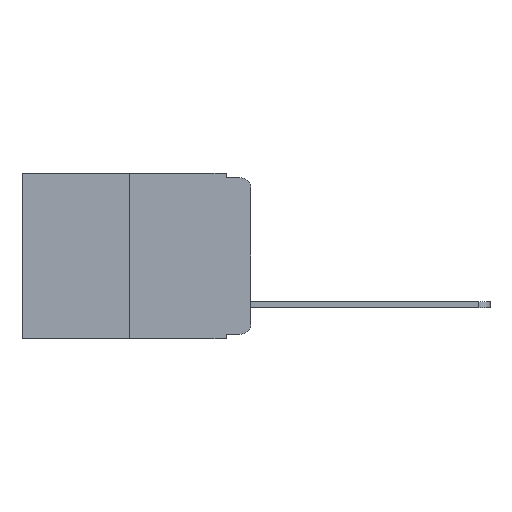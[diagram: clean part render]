
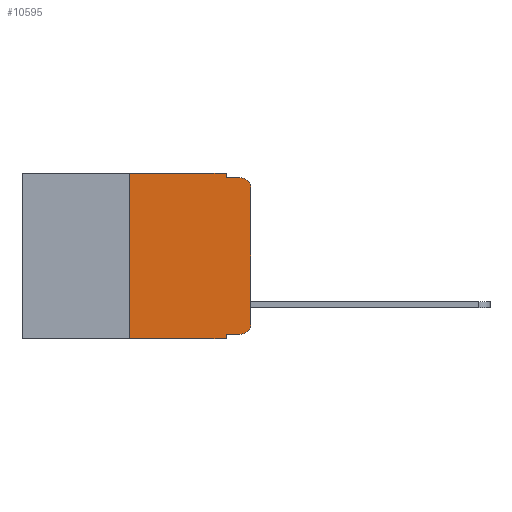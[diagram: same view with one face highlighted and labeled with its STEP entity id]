
A CAD part, left-side view. The second image highlights one B-rep face of the part: STEP entity #10595.
In plain terms, the highlighted planar face has unit normal (-1, 0, 0).
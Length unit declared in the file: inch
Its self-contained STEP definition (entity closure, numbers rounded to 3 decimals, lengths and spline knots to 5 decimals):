
#215 = CIRCLE ( 'NONE', #12082, 0.02 ) ;
#625 = CARTESIAN_POINT ( 'NONE',  ( 0., 0.02, -0.03 ) ) ;
#1014 = VECTOR ( 'NONE', #9177, 39.37008 ) ;
#1016 = CARTESIAN_POINT ( 'NONE',  ( 0., 0.051, -0.343 ) ) ;
#1036 = ORIENTED_EDGE ( 'NONE', *, *, #3050, .T. ) ;
#1070 = ORIENTED_EDGE ( 'NONE', *, *, #10524, .F. ) ;
#1094 = VERTEX_POINT ( 'NONE', #12182 ) ;
#1296 = VERTEX_POINT ( 'NONE', #3679 ) ;
#1349 = AXIS2_PLACEMENT_3D ( 'NONE', #4786, #11981, #3943 ) ;
#1598 = DIRECTION ( 'NONE',  ( 0., 0., -1. ) ) ;
#1734 = VERTEX_POINT ( 'NONE', #9774 ) ;
#1840 = CARTESIAN_POINT ( 'NONE',  ( 0., 0., -0.03 ) ) ;
#2031 = CARTESIAN_POINT ( 'NONE',  ( 0., 0.25, 0. ) ) ;
#2047 = VECTOR ( 'NONE', #7870, 39.37008 ) ;
#2433 = EDGE_CURVE ( 'NONE', #7922, #14541, #15840, .T. ) ;
#2986 = CARTESIAN_POINT ( 'NONE',  ( 0., 0.051, -0.01 ) ) ;
#3050 = EDGE_CURVE ( 'NONE', #1094, #6382, #11726, .T. ) ;
#3128 = VERTEX_POINT ( 'NONE', #5985 ) ;
#3660 = VERTEX_POINT ( 'NONE', #1016 ) ;
#3679 = CARTESIAN_POINT ( 'NONE',  ( 0., 0.02, -0.01 ) ) ;
#3714 = EDGE_CURVE ( 'NONE', #14541, #14164, #4104, .T. ) ;
#3845 = LINE ( 'NONE', #4801, #13199 ) ;
#3943 = DIRECTION ( 'NONE',  ( 0., 0., -1. ) ) ;
#4104 = LINE ( 'NONE', #5399, #11893 ) ;
#4330 = DIRECTION ( 'NONE',  ( -1., 0., 0. ) ) ;
#4376 = CARTESIAN_POINT ( 'NONE',  ( 0., 0., 0. ) ) ;
#4561 = DIRECTION ( 'NONE',  ( 0., -1., 0. ) ) ;
#4786 = CARTESIAN_POINT ( 'NONE',  ( 0., 0.473, 0. ) ) ;
#4801 = CARTESIAN_POINT ( 'NONE',  ( 0., 0.051, 0. ) ) ;
#4833 = ORIENTED_EDGE ( 'NONE', *, *, #2433, .F. ) ;
#5399 = CARTESIAN_POINT ( 'NONE',  ( 0., 0.051, 0. ) ) ;
#5890 = DIRECTION ( 'NONE',  ( 0., 0., -1. ) ) ;
#5968 = EDGE_CURVE ( 'NONE', #8746, #3660, #3845, .T. ) ;
#5985 = CARTESIAN_POINT ( 'NONE',  ( 0., 0.25, -0.343 ) ) ;
#6382 = VERTEX_POINT ( 'NONE', #1840 ) ;
#6638 = AXIS2_PLACEMENT_3D ( 'NONE', #12515, #7379, #16108 ) ;
#6872 = VECTOR ( 'NONE', #4561, 39.37008 ) ;
#6917 = LINE ( 'NONE', #10280, #2047 ) ;
#7094 = CARTESIAN_POINT ( 'NONE',  ( 0., 0.473, 0. ) ) ;
#7379 = DIRECTION ( 'NONE',  ( -1., 0., 0. ) ) ;
#7445 = LINE ( 'NONE', #14098, #12525 ) ;
#7568 = ORIENTED_EDGE ( 'NONE', *, *, #12977, .F. ) ;
#7862 = CARTESIAN_POINT ( 'NONE',  ( 0., 0.25, 0. ) ) ;
#7870 = DIRECTION ( 'NONE',  ( 0., -1., 0. ) ) ;
#7922 = VERTEX_POINT ( 'NONE', #2031 ) ;
#7930 = VECTOR ( 'NONE', #8545, 39.37008 ) ;
#8419 = EDGE_CURVE ( 'NONE', #1734, #1094, #15742, .T. ) ;
#8522 = ORIENTED_EDGE ( 'NONE', *, *, #8419, .T. ) ;
#8545 = DIRECTION ( 'NONE',  ( 0., -1., 0. ) ) ;
#8589 = ORIENTED_EDGE ( 'NONE', *, *, #5968, .F. ) ;
#8746 = VERTEX_POINT ( 'NONE', #14678 ) ;
#8948 = EDGE_LOOP ( 'NONE', ( #1036, #9294, #1070, #12809, #4833, #7568, #10933, #8589, #15335, #8522 ) ) ;
#9177 = DIRECTION ( 'NONE',  ( 0., 0., 1. ) ) ;
#9294 = ORIENTED_EDGE ( 'NONE', *, *, #14126, .T. ) ;
#9774 = CARTESIAN_POINT ( 'NONE',  ( 0., 0.02, -0.333 ) ) ;
#10003 = VECTOR ( 'NONE', #13967, 39.37008 ) ;
#10280 = CARTESIAN_POINT ( 'NONE',  ( 0., 0.051, -0.01 ) ) ;
#10524 = EDGE_CURVE ( 'NONE', #14164, #1296, #6917, .T. ) ;
#10595 = ADVANCED_FACE ( 'NONE', ( #15698 ), #11453, .F. ) ;
#10676 = LINE ( 'NONE', #15976, #7930 ) ;
#10933 = ORIENTED_EDGE ( 'NONE', *, *, #12465, .T. ) ;
#11453 = PLANE ( 'NONE',  #1349 ) ;
#11726 = LINE ( 'NONE', #4376, #1014 ) ;
#11893 = VECTOR ( 'NONE', #1598, 39.37008 ) ;
#11981 = DIRECTION ( 'NONE',  ( 1., 0., 0. ) ) ;
#12082 = AXIS2_PLACEMENT_3D ( 'NONE', #625, #4330, #14282 ) ;
#12182 = CARTESIAN_POINT ( 'NONE',  ( 0., 0., -0.313 ) ) ;
#12465 = EDGE_CURVE ( 'NONE', #3128, #3660, #7445, .T. ) ;
#12515 = CARTESIAN_POINT ( 'NONE',  ( 0., 0.02, -0.313 ) ) ;
#12525 = VECTOR ( 'NONE', #13099, 39.37008 ) ;
#12531 = CARTESIAN_POINT ( 'NONE',  ( 0., 0.051, 0. ) ) ;
#12809 = ORIENTED_EDGE ( 'NONE', *, *, #3714, .F. ) ;
#12977 = EDGE_CURVE ( 'NONE', #3128, #7922, #13569, .T. ) ;
#13099 = DIRECTION ( 'NONE',  ( 0., -1., 0. ) ) ;
#13199 = VECTOR ( 'NONE', #5890, 39.37008 ) ;
#13569 = LINE ( 'NONE', #7862, #10003 ) ;
#13967 = DIRECTION ( 'NONE',  ( 0., 0., 1. ) ) ;
#14098 = CARTESIAN_POINT ( 'NONE',  ( 0., 0.473, -0.343 ) ) ;
#14126 = EDGE_CURVE ( 'NONE', #6382, #1296, #215, .T. ) ;
#14164 = VERTEX_POINT ( 'NONE', #2986 ) ;
#14282 = DIRECTION ( 'NONE',  ( 0., 0., -1. ) ) ;
#14541 = VERTEX_POINT ( 'NONE', #12531 ) ;
#14678 = CARTESIAN_POINT ( 'NONE',  ( 0., 0.051, -0.333 ) ) ;
#15335 = ORIENTED_EDGE ( 'NONE', *, *, #16151, .T. ) ;
#15698 = FACE_OUTER_BOUND ( 'NONE', #8948, .T. ) ;
#15742 = CIRCLE ( 'NONE', #6638, 0.02 ) ;
#15840 = LINE ( 'NONE', #7094, #6872 ) ;
#15976 = CARTESIAN_POINT ( 'NONE',  ( 0., 0.051, -0.333 ) ) ;
#16108 = DIRECTION ( 'NONE',  ( 0., 0., -1. ) ) ;
#16151 = EDGE_CURVE ( 'NONE', #8746, #1734, #10676, .T. ) ;
